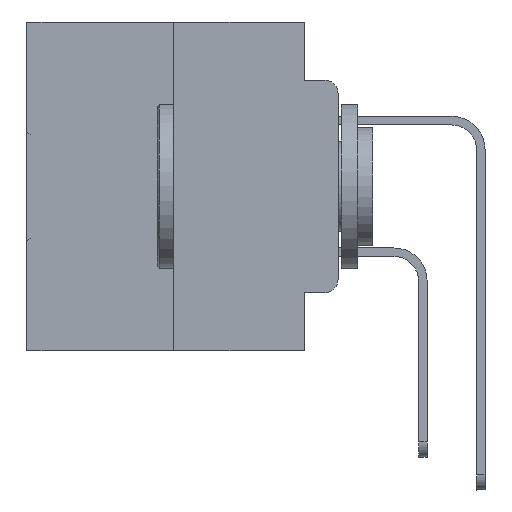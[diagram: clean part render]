
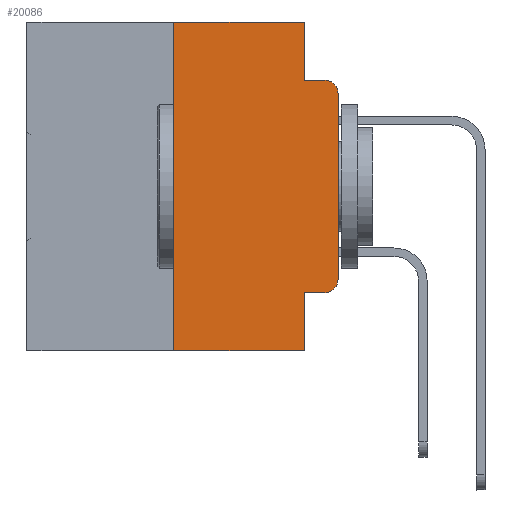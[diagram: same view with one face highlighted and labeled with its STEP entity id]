
A CAD part, left-side view. The second image highlights one B-rep face of the part: STEP entity #20086.
In plain terms, the highlighted planar face has unit normal (-1, 0, 0).
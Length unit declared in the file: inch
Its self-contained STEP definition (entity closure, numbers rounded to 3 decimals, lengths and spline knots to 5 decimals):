
#495 = EDGE_CURVE ( 'NONE', #33553, #11722, #6186, .T. ) ;
#899 = VERTEX_POINT ( 'NONE', #5465 ) ;
#1765 = LINE ( 'NONE', #29240, #9907 ) ;
#1924 = CARTESIAN_POINT ( 'NONE',  ( 0., 0.02, -0.1085 ) ) ;
#2550 = VERTEX_POINT ( 'NONE', #21445 ) ;
#2923 = DIRECTION ( 'NONE',  ( 0., 0., 1. ) ) ;
#3145 = EDGE_LOOP ( 'NONE', ( #9098, #14281, #9546, #11278, #28893, #17244, #11734, #16003, #31798, #5743 ) ) ;
#3482 = DIRECTION ( 'NONE',  ( 0., -1., 0. ) ) ;
#3657 = LINE ( 'NONE', #31683, #24370 ) ;
#4724 = DIRECTION ( 'NONE',  ( 0., 0., -1. ) ) ;
#5465 = CARTESIAN_POINT ( 'NONE',  ( 0., 0.051, -0.4115 ) ) ;
#5743 = ORIENTED_EDGE ( 'NONE', *, *, #34707, .T. ) ;
#6186 = LINE ( 'NONE', #25685, #11759 ) ;
#6564 = CARTESIAN_POINT ( 'NONE',  ( 0., 0.25, -0.5 ) ) ;
#6777 = CARTESIAN_POINT ( 'NONE',  ( 0., 0.25, 0. ) ) ;
#6929 = VERTEX_POINT ( 'NONE', #23077 ) ;
#7461 = CIRCLE ( 'NONE', #31988, 0.02 ) ;
#7495 = CIRCLE ( 'NONE', #12088, 0.02 ) ;
#7914 = CARTESIAN_POINT ( 'NONE',  ( 0., 0.02, -0.4115 ) ) ;
#8951 = VECTOR ( 'NONE', #3482, 39.37008 ) ;
#9098 = ORIENTED_EDGE ( 'NONE', *, *, #24632, .T. ) ;
#9216 = VERTEX_POINT ( 'NONE', #30796 ) ;
#9428 = EDGE_CURVE ( 'NONE', #899, #11722, #25311, .T. ) ;
#9492 = FACE_OUTER_BOUND ( 'NONE', #3145, .T. ) ;
#9546 = ORIENTED_EDGE ( 'NONE', *, *, #11476, .F. ) ;
#9573 = LINE ( 'NONE', #27232, #22243 ) ;
#9907 = VECTOR ( 'NONE', #15984, 39.37008 ) ;
#10551 = EDGE_CURVE ( 'NONE', #9216, #19230, #18561, .T. ) ;
#11017 = CARTESIAN_POINT ( 'NONE',  ( 0., 0.473, 0. ) ) ;
#11278 = ORIENTED_EDGE ( 'NONE', *, *, #10551, .F. ) ;
#11476 = EDGE_CURVE ( 'NONE', #19230, #6929, #3657, .T. ) ;
#11722 = VERTEX_POINT ( 'NONE', #33201 ) ;
#11729 = CARTESIAN_POINT ( 'NONE',  ( 0., 0.473, 0. ) ) ;
#11734 = ORIENTED_EDGE ( 'NONE', *, *, #495, .T. ) ;
#11759 = VECTOR ( 'NONE', #33268, 39.37008 ) ;
#11893 = CARTESIAN_POINT ( 'NONE',  ( 0., 0.02, -0.3915 ) ) ;
#12048 = EDGE_CURVE ( 'NONE', #899, #13063, #1765, .T. ) ;
#12088 = AXIS2_PLACEMENT_3D ( 'NONE', #11893, #30558, #14644 ) ;
#12162 = DIRECTION ( 'NONE',  ( 0., 0., -1. ) ) ;
#13063 = VERTEX_POINT ( 'NONE', #7914 ) ;
#13797 = DIRECTION ( 'NONE',  ( 1., 0., 0. ) ) ;
#14102 = DIRECTION ( 'NONE',  ( 0., 0., 1. ) ) ;
#14281 = ORIENTED_EDGE ( 'NONE', *, *, #16412, .T. ) ;
#14644 = DIRECTION ( 'NONE',  ( 0., 0., -1. ) ) ;
#15194 = LINE ( 'NONE', #30052, #22269 ) ;
#15984 = DIRECTION ( 'NONE',  ( 0., -1., 0. ) ) ;
#16003 = ORIENTED_EDGE ( 'NONE', *, *, #9428, .F. ) ;
#16412 = EDGE_CURVE ( 'NONE', #29361, #6929, #7461, .T. ) ;
#16588 = EDGE_CURVE ( 'NONE', #33553, #24873, #9573, .T. ) ;
#17244 = ORIENTED_EDGE ( 'NONE', *, *, #16588, .F. ) ;
#18561 = LINE ( 'NONE', #30710, #30188 ) ;
#19230 = VERTEX_POINT ( 'NONE', #23451 ) ;
#20086 = ADVANCED_FACE ( 'NONE', ( #9492 ), #29767, .F. ) ;
#20966 = DIRECTION ( 'NONE',  ( -1., 0., 0. ) ) ;
#21154 = CARTESIAN_POINT ( 'NONE',  ( 0., 0.051, 0. ) ) ;
#21445 = CARTESIAN_POINT ( 'NONE',  ( 0., 0., -0.3915 ) ) ;
#22243 = VECTOR ( 'NONE', #2923, 39.37008 ) ;
#22269 = VECTOR ( 'NONE', #14102, 39.37008 ) ;
#22807 = VECTOR ( 'NONE', #23836, 39.37008 ) ;
#23077 = CARTESIAN_POINT ( 'NONE',  ( 0., 0.02, -0.0885 ) ) ;
#23418 = CARTESIAN_POINT ( 'NONE',  ( 0., 0., -0.1085 ) ) ;
#23451 = CARTESIAN_POINT ( 'NONE',  ( 0., 0.051, -0.0885 ) ) ;
#23836 = DIRECTION ( 'NONE',  ( 0., 0., -1. ) ) ;
#24370 = VECTOR ( 'NONE', #34340, 39.37008 ) ;
#24632 = EDGE_CURVE ( 'NONE', #2550, #29361, #15194, .T. ) ;
#24873 = VERTEX_POINT ( 'NONE', #6777 ) ;
#25311 = LINE ( 'NONE', #21154, #22807 ) ;
#25685 = CARTESIAN_POINT ( 'NONE',  ( 0., 0.473, -0.5 ) ) ;
#27232 = CARTESIAN_POINT ( 'NONE',  ( 0., 0.25, 0. ) ) ;
#28893 = ORIENTED_EDGE ( 'NONE', *, *, #31586, .F. ) ;
#29240 = CARTESIAN_POINT ( 'NONE',  ( 0., 0.051, -0.4115 ) ) ;
#29361 = VERTEX_POINT ( 'NONE', #23418 ) ;
#29767 = PLANE ( 'NONE',  #34065 ) ;
#30052 = CARTESIAN_POINT ( 'NONE',  ( 0., 0., 0. ) ) ;
#30188 = VECTOR ( 'NONE', #12162, 39.37008 ) ;
#30558 = DIRECTION ( 'NONE',  ( -1., 0., 0. ) ) ;
#30710 = CARTESIAN_POINT ( 'NONE',  ( 0., 0.051, 0. ) ) ;
#30796 = CARTESIAN_POINT ( 'NONE',  ( 0., 0.051, 0. ) ) ;
#31192 = LINE ( 'NONE', #11729, #8951 ) ;
#31586 = EDGE_CURVE ( 'NONE', #24873, #9216, #31192, .T. ) ;
#31683 = CARTESIAN_POINT ( 'NONE',  ( 0., 0.051, -0.0885 ) ) ;
#31798 = ORIENTED_EDGE ( 'NONE', *, *, #12048, .T. ) ;
#31988 = AXIS2_PLACEMENT_3D ( 'NONE', #1924, #20966, #4724 ) ;
#32418 = DIRECTION ( 'NONE',  ( 0., 0., -1. ) ) ;
#33201 = CARTESIAN_POINT ( 'NONE',  ( 0., 0.051, -0.5 ) ) ;
#33268 = DIRECTION ( 'NONE',  ( 0., -1., 0. ) ) ;
#33553 = VERTEX_POINT ( 'NONE', #6564 ) ;
#34065 = AXIS2_PLACEMENT_3D ( 'NONE', #11017, #13797, #32418 ) ;
#34340 = DIRECTION ( 'NONE',  ( 0., -1., 0. ) ) ;
#34707 = EDGE_CURVE ( 'NONE', #13063, #2550, #7495, .T. ) ;
